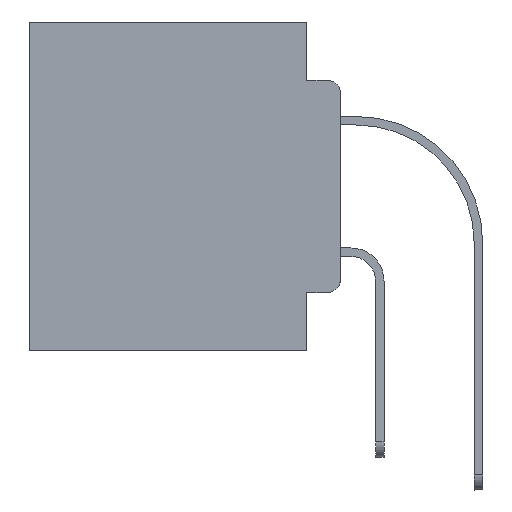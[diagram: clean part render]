
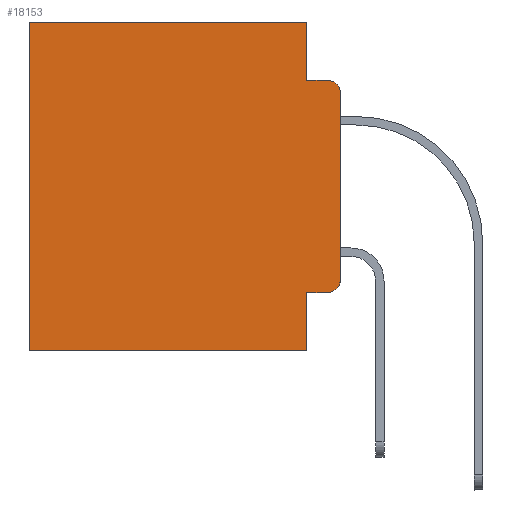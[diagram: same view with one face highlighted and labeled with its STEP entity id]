
A CAD part, left-side view. The second image highlights one B-rep face of the part: STEP entity #18153.
In plain terms, the highlighted planar face has unit normal (-1, 0, 0).
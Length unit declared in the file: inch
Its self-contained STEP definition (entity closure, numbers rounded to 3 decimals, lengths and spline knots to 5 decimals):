
#104 = VECTOR ( 'NONE', #28344, 39.37008 ) ;
#1297 = ORIENTED_EDGE ( 'NONE', *, *, #21452, .T. ) ;
#1461 = LINE ( 'NONE', #27583, #26011 ) ;
#1782 = DIRECTION ( 'NONE',  ( 0., -1., 0. ) ) ;
#1783 = DIRECTION ( 'NONE',  ( 0., 1., 0. ) ) ;
#1817 = DIRECTION ( 'NONE',  ( 0., 0., -1. ) ) ;
#2162 = AXIS2_PLACEMENT_3D ( 'NONE', #30268, #15883, #1817 ) ;
#2315 = CARTESIAN_POINT ( 'NONE',  ( 0.298, 0.02, -0.3915 ) ) ;
#2618 = CARTESIAN_POINT ( 'NONE',  ( 0.298, 0.051, -0.5 ) ) ;
#2702 = CARTESIAN_POINT ( 'NONE',  ( 0.298, 0.051, -0.4115 ) ) ;
#3332 = VECTOR ( 'NONE', #25763, 39.37008 ) ;
#3549 = PLANE ( 'NONE',  #2162 ) ;
#4131 = DIRECTION ( 'NONE',  ( 0., 0., -1. ) ) ;
#4468 = CARTESIAN_POINT ( 'NONE',  ( 0.298, 0., -0.3915 ) ) ;
#5189 = EDGE_CURVE ( 'NONE', #16156, #29478, #9200, .T. ) ;
#5339 = LINE ( 'NONE', #2702, #20382 ) ;
#5655 = CARTESIAN_POINT ( 'NONE',  ( 0.298, 0.051, 0. ) ) ;
#5992 = ORIENTED_EDGE ( 'NONE', *, *, #6541, .T. ) ;
#5998 = CARTESIAN_POINT ( 'NONE',  ( 0.298, 0.051, -0.0885 ) ) ;
#6075 = EDGE_CURVE ( 'NONE', #25999, #7759, #17347, .T. ) ;
#6165 = DIRECTION ( 'NONE',  ( 0., 0., -1. ) ) ;
#6541 = EDGE_CURVE ( 'NONE', #16082, #29975, #28212, .T. ) ;
#7376 = AXIS2_PLACEMENT_3D ( 'NONE', #28003, #14081, #13766 ) ;
#7759 = VERTEX_POINT ( 'NONE', #23141 ) ;
#8105 = FACE_OUTER_BOUND ( 'NONE', #11448, .T. ) ;
#8676 = CARTESIAN_POINT ( 'NONE',  ( 0.298, 0.051, 0. ) ) ;
#9200 = LINE ( 'NONE', #16384, #3332 ) ;
#9649 = CARTESIAN_POINT ( 'NONE',  ( 0.298, 0.02, -0.4115 ) ) ;
#10138 = EDGE_CURVE ( 'NONE', #21626, #29015, #11970, .T. ) ;
#11448 = EDGE_LOOP ( 'NONE', ( #25713, #30318, #30101, #29691, #23232, #29207, #16754, #14320, #1297, #5992 ) ) ;
#11970 = LINE ( 'NONE', #21513, #16526 ) ;
#12134 = DIRECTION ( 'NONE',  ( 0., 0., -1. ) ) ;
#13766 = DIRECTION ( 'NONE',  ( 0., 0., -1. ) ) ;
#13801 = CARTESIAN_POINT ( 'NONE',  ( 0.298, 0.473, 0. ) ) ;
#14081 = DIRECTION ( 'NONE',  ( -1., 0., 0. ) ) ;
#14121 = CARTESIAN_POINT ( 'NONE',  ( 0.298, 0., -0.1085 ) ) ;
#14320 = ORIENTED_EDGE ( 'NONE', *, *, #23061, .F. ) ;
#15085 = LINE ( 'NONE', #5998, #20000 ) ;
#15833 = LINE ( 'NONE', #8676, #19374 ) ;
#15883 = DIRECTION ( 'NONE',  ( 1., 0., 0. ) ) ;
#16082 = VERTEX_POINT ( 'NONE', #9649 ) ;
#16156 = VERTEX_POINT ( 'NONE', #2618 ) ;
#16384 = CARTESIAN_POINT ( 'NONE',  ( 0.298, 0., -0.5 ) ) ;
#16526 = VECTOR ( 'NONE', #12134, 39.37008 ) ;
#16754 = ORIENTED_EDGE ( 'NONE', *, *, #5189, .F. ) ;
#16883 = EDGE_CURVE ( 'NONE', #25999, #29975, #30548, .T. ) ;
#16887 = CARTESIAN_POINT ( 'NONE',  ( 0.298, 0.051, -0.0885 ) ) ;
#17173 = DIRECTION ( 'NONE',  ( 0., 0., -1. ) ) ;
#17347 = CIRCLE ( 'NONE', #7376, 0.02 ) ;
#17934 = VECTOR ( 'NONE', #1783, 39.37008 ) ;
#18153 = ADVANCED_FACE ( 'NONE', ( #8105 ), #3549, .F. ) ;
#18209 = LINE ( 'NONE', #27728, #17934 ) ;
#18586 = CARTESIAN_POINT ( 'NONE',  ( 0.298, 0.473, -0.5 ) ) ;
#19374 = VECTOR ( 'NONE', #4131, 39.37008 ) ;
#20000 = VECTOR ( 'NONE', #1782, 39.37008 ) ;
#20382 = VECTOR ( 'NONE', #29253, 39.37008 ) ;
#21452 = EDGE_CURVE ( 'NONE', #30338, #16082, #5339, .T. ) ;
#21513 = CARTESIAN_POINT ( 'NONE',  ( 0.298, 0.051, 0. ) ) ;
#21626 = VERTEX_POINT ( 'NONE', #5655 ) ;
#23061 = EDGE_CURVE ( 'NONE', #30338, #16156, #15833, .T. ) ;
#23141 = CARTESIAN_POINT ( 'NONE',  ( 0.298, 0.02, -0.0885 ) ) ;
#23232 = ORIENTED_EDGE ( 'NONE', *, *, #24321, .T. ) ;
#24321 = EDGE_CURVE ( 'NONE', #21626, #30370, #18209, .T. ) ;
#25713 = ORIENTED_EDGE ( 'NONE', *, *, #16883, .F. ) ;
#25752 = EDGE_CURVE ( 'NONE', #30370, #29478, #1461, .T. ) ;
#25763 = DIRECTION ( 'NONE',  ( 0., 1., 0. ) ) ;
#25999 = VERTEX_POINT ( 'NONE', #14121 ) ;
#26011 = VECTOR ( 'NONE', #6165, 39.37008 ) ;
#27105 = EDGE_CURVE ( 'NONE', #29015, #7759, #15085, .T. ) ;
#27583 = CARTESIAN_POINT ( 'NONE',  ( 0.298, 0.473, 0. ) ) ;
#27728 = CARTESIAN_POINT ( 'NONE',  ( 0.298, 0., 0. ) ) ;
#28003 = CARTESIAN_POINT ( 'NONE',  ( 0.298, 0.02, -0.1085 ) ) ;
#28212 = CIRCLE ( 'NONE', #29714, 0.02 ) ;
#28344 = DIRECTION ( 'NONE',  ( 0., 0., -1. ) ) ;
#28732 = DIRECTION ( 'NONE',  ( -1., 0., 0. ) ) ;
#29015 = VERTEX_POINT ( 'NONE', #16887 ) ;
#29207 = ORIENTED_EDGE ( 'NONE', *, *, #25752, .T. ) ;
#29253 = DIRECTION ( 'NONE',  ( 0., -1., 0. ) ) ;
#29478 = VERTEX_POINT ( 'NONE', #18586 ) ;
#29691 = ORIENTED_EDGE ( 'NONE', *, *, #10138, .F. ) ;
#29714 = AXIS2_PLACEMENT_3D ( 'NONE', #2315, #28732, #17173 ) ;
#29975 = VERTEX_POINT ( 'NONE', #4468 ) ;
#30101 = ORIENTED_EDGE ( 'NONE', *, *, #27105, .F. ) ;
#30268 = CARTESIAN_POINT ( 'NONE',  ( 0.298, 0., 0. ) ) ;
#30318 = ORIENTED_EDGE ( 'NONE', *, *, #6075, .T. ) ;
#30338 = VERTEX_POINT ( 'NONE', #30833 ) ;
#30370 = VERTEX_POINT ( 'NONE', #13801 ) ;
#30548 = LINE ( 'NONE', #30692, #104 ) ;
#30692 = CARTESIAN_POINT ( 'NONE',  ( 0.298, 0., 0. ) ) ;
#30833 = CARTESIAN_POINT ( 'NONE',  ( 0.298, 0.051, -0.4115 ) ) ;
